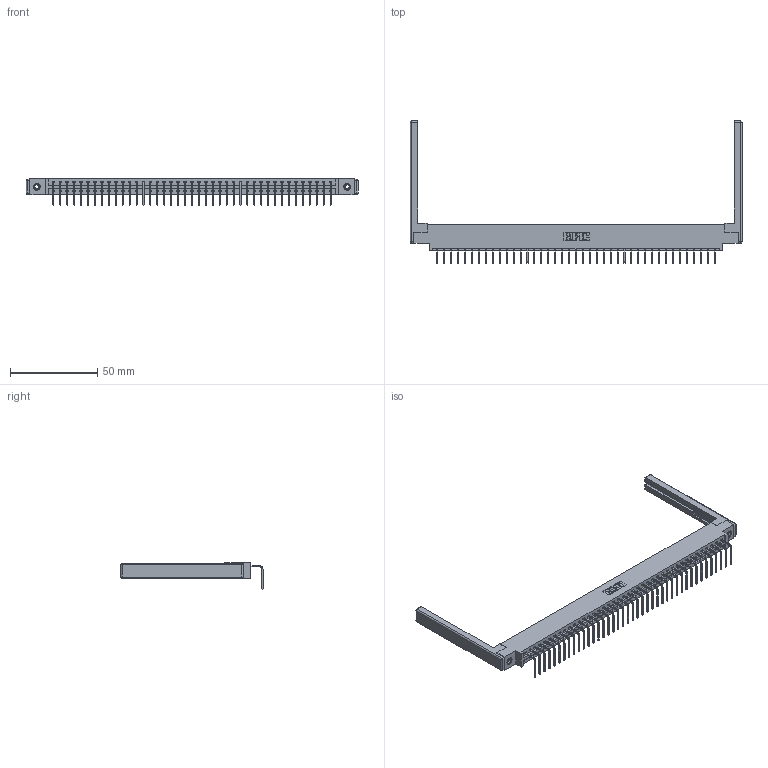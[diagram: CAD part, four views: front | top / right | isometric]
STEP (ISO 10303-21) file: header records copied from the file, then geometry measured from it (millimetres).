
FILE_DESCRIPTION (( 'STEP AP203' ), '1' );
FILE_NAME ('337-041-558-668.STEP', '2019-10-07T15:18:18', ( '' ), ( '' ), 'SwSTEP 2.0', 'SolidWorks 2016', '' );
FILE_SCHEMA (( 'CONFIG_CONTROL_DESIGN' ));
Length unit declared in the file: inch
Products named in the file (5): 337-041-558-668; 345-292-001_558 Tail - 2; 337 Part_0.170 Offset - 0.156 Dia-TI; 307-220-068; 345-250-001_345-250-001-102
Assembly tree (46 placements, depth 2):
  337-041-558-668
    337 Part_0.170 Offset - 0.156 Dia-TI
    345-292-001_558 Tail - 2  x41
    345-250-001_345-250-001-102  x2
    307-220-068  x2
Bounding box: 189.89 x 81.22 x 15.37 mm (x, y, z)
Volume: 24133.7 mm3; surface area: 25423.7 mm2
Topology: 46 solids, 46 shells, 2896 faces, 8667 edges, 5702 vertices
Faces by surface type: plane 2130, cylinder 742, cone 12, sphere 8, torus 4
Entity records: 33582 total; most frequent: CARTESIAN_POINT 5806, ORIENTED_EDGE 5772, DIRECTION 4962, EDGE_CURVE 2886, LINE 2708, VECTOR 2708, VERTEX_POINT 1914, AXIS2_PLACEMENT_3D 1127
